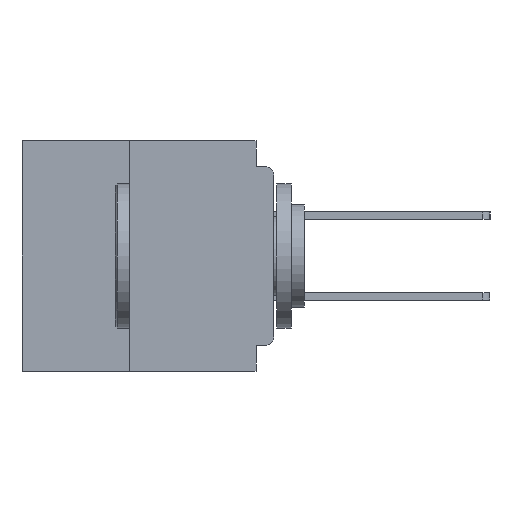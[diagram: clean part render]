
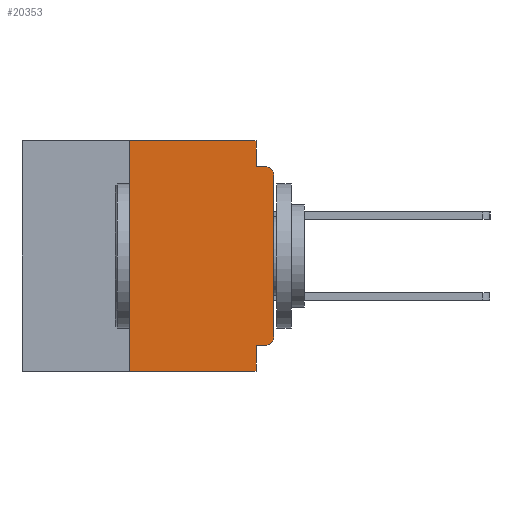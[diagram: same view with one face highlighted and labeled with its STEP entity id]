
A CAD part, left-side view. The second image highlights one B-rep face of the part: STEP entity #20353.
In plain terms, the highlighted planar face has unit normal (-1, 0, 0).
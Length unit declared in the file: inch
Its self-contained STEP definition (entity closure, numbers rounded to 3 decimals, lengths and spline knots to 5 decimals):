
#570 = CARTESIAN_POINT ( 'NONE',  ( 0., 0., -0.06 ) ) ;
#1386 = CARTESIAN_POINT ( 'NONE',  ( 0., 0.031, -0.4 ) ) ;
#1909 = LINE ( 'NONE', #35038, #11827 ) ;
#2281 = VERTEX_POINT ( 'NONE', #51418 ) ;
#2391 = CARTESIAN_POINT ( 'NONE',  ( 0., 0.25, -0.4 ) ) ;
#3333 = AXIS2_PLACEMENT_3D ( 'NONE', #19299, #19217, #19115 ) ;
#3414 = EDGE_CURVE ( 'NONE', #36442, #34158, #6808, .T. ) ;
#5684 = CARTESIAN_POINT ( 'NONE',  ( 0., 0.031, 0. ) ) ;
#6808 = CIRCLE ( 'NONE', #3333, 0.015 ) ;
#6871 = CARTESIAN_POINT ( 'NONE',  ( 0., 0., -0.355 ) ) ;
#8290 = DIRECTION ( 'NONE',  ( 0., 0., -1. ) ) ;
#8327 = ORIENTED_EDGE ( 'NONE', *, *, #52339, .F. ) ;
#8801 = ORIENTED_EDGE ( 'NONE', *, *, #14775, .T. ) ;
#10475 = VERTEX_POINT ( 'NONE', #23090 ) ;
#10613 = CARTESIAN_POINT ( 'NONE',  ( 0., 0.015, -0.045 ) ) ;
#11827 = VECTOR ( 'NONE', #43366, 39.37008 ) ;
#13368 = VERTEX_POINT ( 'NONE', #1386 ) ;
#13381 = EDGE_CURVE ( 'NONE', #10475, #33965, #21943, .T. ) ;
#13552 = ORIENTED_EDGE ( 'NONE', *, *, #3414, .T. ) ;
#13920 = ORIENTED_EDGE ( 'NONE', *, *, #47148, .F. ) ;
#14775 = EDGE_CURVE ( 'NONE', #2281, #36442, #19190, .T. ) ;
#14820 = ORIENTED_EDGE ( 'NONE', *, *, #18517, .F. ) ;
#18362 = ORIENTED_EDGE ( 'NONE', *, *, #13381, .F. ) ;
#18517 = EDGE_CURVE ( 'NONE', #33134, #53313, #49401, .T. ) ;
#18989 = CARTESIAN_POINT ( 'NONE',  ( 0., 0.031, -0.355 ) ) ;
#19115 = DIRECTION ( 'NONE',  ( 0., 0., -1. ) ) ;
#19190 = LINE ( 'NONE', #43841, #50997 ) ;
#19197 = VECTOR ( 'NONE', #8290, 39.37008 ) ;
#19217 = DIRECTION ( 'NONE',  ( -1., 0., 0. ) ) ;
#19299 = CARTESIAN_POINT ( 'NONE',  ( 0., 0.015, -0.06 ) ) ;
#19416 = DIRECTION ( 'NONE',  ( 0., -1., 0. ) ) ;
#19472 = ORIENTED_EDGE ( 'NONE', *, *, #31111, .F. ) ;
#19502 = ORIENTED_EDGE ( 'NONE', *, *, #52109, .T. ) ;
#20353 = ADVANCED_FACE ( 'NONE', ( #53697 ), #40666, .F. ) ;
#20770 = LINE ( 'NONE', #44560, #52600 ) ;
#21943 = LINE ( 'NONE', #5684, #42734 ) ;
#22297 = EDGE_LOOP ( 'NONE', ( #8801, #13552, #13920, #18362, #19472, #23259, #25010, #8327, #14820, #19502 ) ) ;
#23090 = CARTESIAN_POINT ( 'NONE',  ( 0., 0.031, 0. ) ) ;
#23259 = ORIENTED_EDGE ( 'NONE', *, *, #37931, .F. ) ;
#23639 = DIRECTION ( 'NONE',  ( -1., 0., 0. ) ) ;
#25010 = ORIENTED_EDGE ( 'NONE', *, *, #48736, .T. ) ;
#27084 = AXIS2_PLACEMENT_3D ( 'NONE', #36492, #48786, #44794 ) ;
#27347 = VECTOR ( 'NONE', #32063, 39.37008 ) ;
#27350 = CARTESIAN_POINT ( 'NONE',  ( 0., 0.25, -0.4 ) ) ;
#27639 = CIRCLE ( 'NONE', #37053, 0.015 ) ;
#28623 = VECTOR ( 'NONE', #31561, 39.37008 ) ;
#29088 = CARTESIAN_POINT ( 'NONE',  ( 0., 0.031, -0.4 ) ) ;
#31111 = EDGE_CURVE ( 'NONE', #34208, #10475, #44245, .T. ) ;
#31561 = DIRECTION ( 'NONE',  ( 0., 0., 1. ) ) ;
#32063 = DIRECTION ( 'NONE',  ( 0., 1., 0. ) ) ;
#33134 = VERTEX_POINT ( 'NONE', #53836 ) ;
#33965 = VERTEX_POINT ( 'NONE', #33978 ) ;
#33978 = CARTESIAN_POINT ( 'NONE',  ( 0., 0.031, -0.045 ) ) ;
#34158 = VERTEX_POINT ( 'NONE', #10613 ) ;
#34208 = VERTEX_POINT ( 'NONE', #39930 ) ;
#35038 = CARTESIAN_POINT ( 'NONE',  ( 0., 0., -0.045 ) ) ;
#36442 = VERTEX_POINT ( 'NONE', #570 ) ;
#36492 = CARTESIAN_POINT ( 'NONE',  ( 0., 0.437, 0. ) ) ;
#37053 = AXIS2_PLACEMENT_3D ( 'NONE', #48488, #23639, #52683 ) ;
#37931 = EDGE_CURVE ( 'NONE', #40446, #34208, #50677, .T. ) ;
#39930 = CARTESIAN_POINT ( 'NONE',  ( 0., 0.25, 0. ) ) ;
#40446 = VERTEX_POINT ( 'NONE', #2391 ) ;
#40666 = PLANE ( 'NONE',  #27084 ) ;
#42734 = VECTOR ( 'NONE', #51337, 39.37008 ) ;
#43366 = DIRECTION ( 'NONE',  ( 0., -1., 0. ) ) ;
#43841 = CARTESIAN_POINT ( 'NONE',  ( 0., 0., 0. ) ) ;
#44245 = LINE ( 'NONE', #44266, #45525 ) ;
#44266 = CARTESIAN_POINT ( 'NONE',  ( 0., 0.437, 0. ) ) ;
#44560 = CARTESIAN_POINT ( 'NONE',  ( 0., 0.437, -0.4 ) ) ;
#44794 = DIRECTION ( 'NONE',  ( 0., 0., -1. ) ) ;
#45525 = VECTOR ( 'NONE', #19416, 39.37008 ) ;
#47148 = EDGE_CURVE ( 'NONE', #33965, #34158, #1909, .T. ) ;
#47966 = DIRECTION ( 'NONE',  ( 0., 0., 1. ) ) ;
#48488 = CARTESIAN_POINT ( 'NONE',  ( 0., 0.015, -0.34 ) ) ;
#48711 = DIRECTION ( 'NONE',  ( 0., -1., 0. ) ) ;
#48736 = EDGE_CURVE ( 'NONE', #40446, #13368, #20770, .T. ) ;
#48786 = DIRECTION ( 'NONE',  ( 1., 0., 0. ) ) ;
#49401 = LINE ( 'NONE', #6871, #27347 ) ;
#50677 = LINE ( 'NONE', #27350, #28623 ) ;
#50997 = VECTOR ( 'NONE', #47966, 39.37008 ) ;
#51337 = DIRECTION ( 'NONE',  ( 0., 0., -1. ) ) ;
#51418 = CARTESIAN_POINT ( 'NONE',  ( 0., 0., -0.34 ) ) ;
#52109 = EDGE_CURVE ( 'NONE', #33134, #2281, #27639, .T. ) ;
#52314 = LINE ( 'NONE', #29088, #19197 ) ;
#52339 = EDGE_CURVE ( 'NONE', #53313, #13368, #52314, .T. ) ;
#52600 = VECTOR ( 'NONE', #48711, 39.37008 ) ;
#52683 = DIRECTION ( 'NONE',  ( 0., 0., -1. ) ) ;
#53313 = VERTEX_POINT ( 'NONE', #18989 ) ;
#53697 = FACE_OUTER_BOUND ( 'NONE', #22297, .T. ) ;
#53836 = CARTESIAN_POINT ( 'NONE',  ( 0., 0.015, -0.355 ) ) ;
